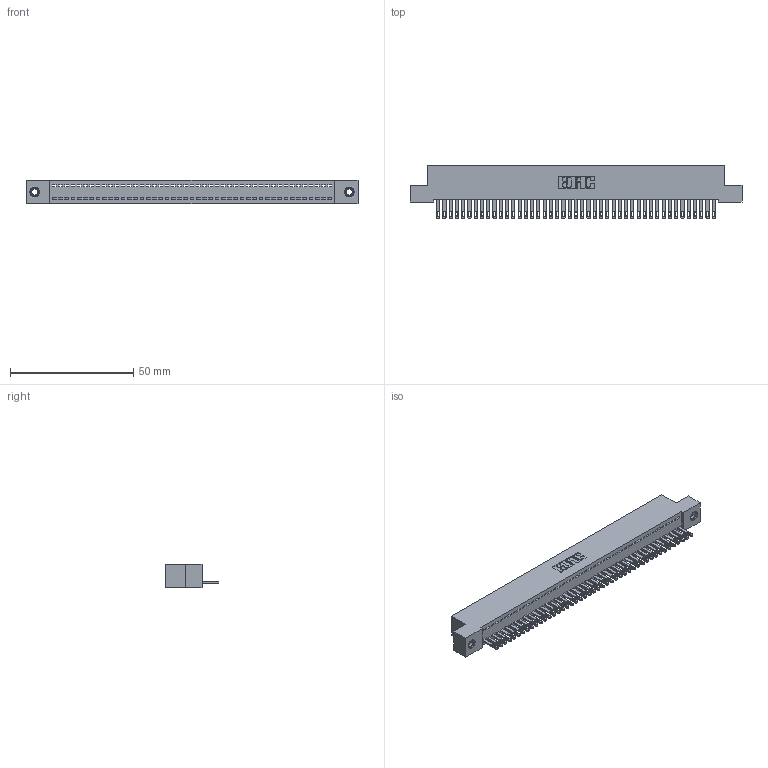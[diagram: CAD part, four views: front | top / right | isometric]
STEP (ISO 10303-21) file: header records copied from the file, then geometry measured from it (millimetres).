
FILE_DESCRIPTION (( 'STEP AP203' ), '1' );
FILE_NAME ('342-045-500-107.STEP', '2018-08-12T15:11:21', ( '' ), ( '' ), 'SwSTEP 2.0', 'SolidWorks 2016', '' );
FILE_SCHEMA (( 'CONFIG_CONTROL_DESIGN' ));
Length unit declared in the file: inch
Products named in the file (4): 342 Part_TI; 345-292-001_345-293-100; 345-250-001_345-250-005-103; 342-045-500-107
Assembly tree (48 placements, depth 2):
  342-045-500-107
    342 Part_TI
    345-292-001_345-293-100  x45
    345-250-001_345-250-005-103  x2
Bounding box: 134.62 x 21.85 x 9.4 mm (x, y, z)
Volume: 11829.7 mm3; surface area: 17548.2 mm2
Topology: 48 solids, 48 shells, 2600 faces, 7995 edges, 5322 vertices
Faces by surface type: plane 1718, cylinder 866, cone 12, torus 4
Entity records: 28106 total; most frequent: CARTESIAN_POINT 4828, ORIENTED_EDGE 4802, DIRECTION 4101, EDGE_CURVE 2401, VECTOR 2249, LINE 2249, VERTEX_POINT 1596, AXIS2_PLACEMENT_3D 926
